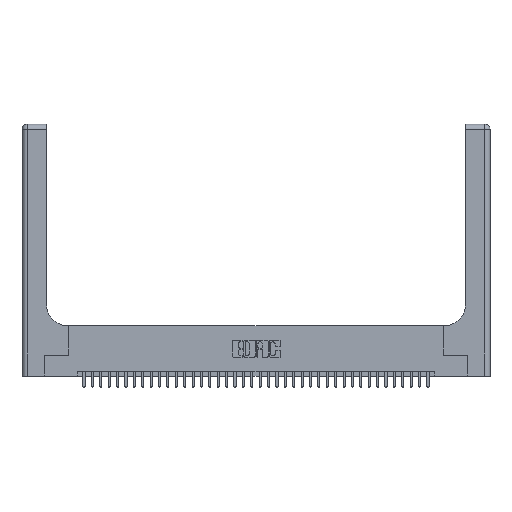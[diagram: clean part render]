
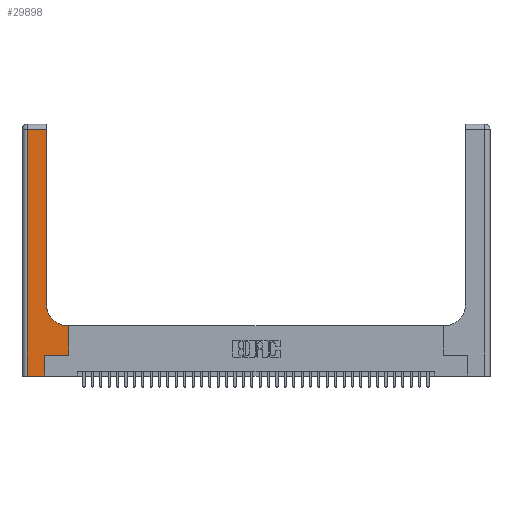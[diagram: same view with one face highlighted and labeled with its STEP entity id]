
A CAD part, top view. The second image highlights one B-rep face of the part: STEP entity #29898.
In plain terms, the highlighted planar face has unit normal (0, 0, 1).
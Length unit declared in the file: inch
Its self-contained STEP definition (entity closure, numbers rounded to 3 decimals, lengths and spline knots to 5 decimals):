
#267 = ORIENTED_EDGE ( 'NONE', *, *, #32464, .T. ) ;
#625 = DIRECTION ( 'NONE',  ( 0., -1., 0. ) ) ;
#707 = VERTEX_POINT ( 'NONE', #28314 ) ;
#1085 = LINE ( 'NONE', #29768, #14064 ) ;
#2202 = CARTESIAN_POINT ( 'NONE',  ( 0.2915, 3., 0.37 ) ) ;
#2213 = DIRECTION ( 'NONE',  ( -1., 0., 0. ) ) ;
#2572 = AXIS2_PLACEMENT_3D ( 'NONE', #37485, #19864, #2213 ) ;
#3035 = VECTOR ( 'NONE', #11251, 39.37008 ) ;
#3456 = LINE ( 'NONE', #30821, #24136 ) ;
#3548 = LINE ( 'NONE', #33597, #28807 ) ;
#3603 = VERTEX_POINT ( 'NONE', #14935 ) ;
#3703 = AXIS2_PLACEMENT_3D ( 'NONE', #13306, #33821, #16253 ) ;
#4311 = CARTESIAN_POINT ( 'NONE',  ( 0.269, 0., 0.37 ) ) ;
#5079 = EDGE_CURVE ( 'NONE', #17319, #26706, #3456, .T. ) ;
#5212 = DIRECTION ( 'NONE',  ( 0., 1., 0. ) ) ;
#5476 = ORIENTED_EDGE ( 'NONE', *, *, #27689, .T. ) ;
#7870 = LINE ( 'NONE', #21252, #30346 ) ;
#9559 = ORIENTED_EDGE ( 'NONE', *, *, #33036, .T. ) ;
#10577 = DIRECTION ( 'NONE',  ( 1., 0., 0. ) ) ;
#11113 = VERTEX_POINT ( 'NONE', #31194 ) ;
#11251 = DIRECTION ( 'NONE',  ( -1., 0., 0. ) ) ;
#12202 = VERTEX_POINT ( 'NONE', #25730 ) ;
#12264 = VERTEX_POINT ( 'NONE', #17301 ) ;
#13306 = CARTESIAN_POINT ( 'NONE',  ( 0.5415, 0.85, 0.37 ) ) ;
#14064 = VECTOR ( 'NONE', #15214, 39.37008 ) ;
#14437 = CARTESIAN_POINT ( 'NONE',  ( 0.06, 0., 0.37 ) ) ;
#14837 = EDGE_CURVE ( 'NONE', #19416, #22177, #33388, .T. ) ;
#14935 = CARTESIAN_POINT ( 'NONE',  ( 0.5585, 0.6, 0.37 ) ) ;
#15214 = DIRECTION ( 'NONE',  ( -1., 0., 0. ) ) ;
#15596 = VECTOR ( 'NONE', #15685, 39.37008 ) ;
#15685 = DIRECTION ( 'NONE',  ( 0., 1., 0. ) ) ;
#16253 = DIRECTION ( 'NONE',  ( 1., 0., 0. ) ) ;
#16588 = EDGE_CURVE ( 'NONE', #707, #19416, #37351, .T. ) ;
#16941 = PLANE ( 'NONE',  #2572 ) ;
#17301 = CARTESIAN_POINT ( 'NONE',  ( 0.269, 0.25, 0.37 ) ) ;
#17319 = VERTEX_POINT ( 'NONE', #14437 ) ;
#18132 = EDGE_CURVE ( 'NONE', #12202, #707, #29804, .T. ) ;
#18505 = CARTESIAN_POINT ( 'NONE',  ( 0.5585, 0.25, 0.37 ) ) ;
#18784 = ORIENTED_EDGE ( 'NONE', *, *, #37670, .T. ) ;
#19326 = CARTESIAN_POINT ( 'NONE',  ( 0.269, 0.25, 0.37 ) ) ;
#19416 = VERTEX_POINT ( 'NONE', #27663 ) ;
#19864 = DIRECTION ( 'NONE',  ( 0., 0., -1. ) ) ;
#21252 = CARTESIAN_POINT ( 'NONE',  ( 0.06, 3., 0.37 ) ) ;
#21465 = ORIENTED_EDGE ( 'NONE', *, *, #5079, .T. ) ;
#22177 = VERTEX_POINT ( 'NONE', #37873 ) ;
#23357 = LINE ( 'NONE', #18505, #15596 ) ;
#23522 = VECTOR ( 'NONE', #5212, 39.37008 ) ;
#24136 = VECTOR ( 'NONE', #27965, 39.37008 ) ;
#25730 = CARTESIAN_POINT ( 'NONE',  ( 0.5415, 0.6, 0.37 ) ) ;
#26331 = EDGE_LOOP ( 'NONE', ( #28880, #33809, #27396, #21465, #267, #9559, #18784, #5476, #35522 ) ) ;
#26706 = VERTEX_POINT ( 'NONE', #4311 ) ;
#27396 = ORIENTED_EDGE ( 'NONE', *, *, #36516, .T. ) ;
#27663 = CARTESIAN_POINT ( 'NONE',  ( 0.2915, 2.94, 0.37 ) ) ;
#27689 = EDGE_CURVE ( 'NONE', #3603, #12202, #1085, .T. ) ;
#27965 = DIRECTION ( 'NONE',  ( 1., 0., 0. ) ) ;
#28314 = CARTESIAN_POINT ( 'NONE',  ( 0.2915, 0.85, 0.37 ) ) ;
#28807 = VECTOR ( 'NONE', #36570, 39.37008 ) ;
#28880 = ORIENTED_EDGE ( 'NONE', *, *, #16588, .T. ) ;
#29768 = CARTESIAN_POINT ( 'NONE',  ( 0.2915, 0.6, 0.37 ) ) ;
#29804 = CIRCLE ( 'NONE', #3703, 0.25 ) ;
#29898 = ADVANCED_FACE ( 'NONE', ( #36831 ), #16941, .F. ) ;
#30148 = VECTOR ( 'NONE', #10577, 39.37008 ) ;
#30346 = VECTOR ( 'NONE', #625, 39.37008 ) ;
#30821 = CARTESIAN_POINT ( 'NONE',  ( 0., 0., 0.37 ) ) ;
#31194 = CARTESIAN_POINT ( 'NONE',  ( 0.5585, 0.25, 0.37 ) ) ;
#31774 = CARTESIAN_POINT ( 'NONE',  ( 0., 2.94, 0.37 ) ) ;
#32464 = EDGE_CURVE ( 'NONE', #26706, #12264, #3548, .T. ) ;
#33036 = EDGE_CURVE ( 'NONE', #12264, #11113, #38022, .T. ) ;
#33388 = LINE ( 'NONE', #31774, #3035 ) ;
#33597 = CARTESIAN_POINT ( 'NONE',  ( 0.269, 0., 0.37 ) ) ;
#33809 = ORIENTED_EDGE ( 'NONE', *, *, #14837, .T. ) ;
#33821 = DIRECTION ( 'NONE',  ( 0., 0., -1. ) ) ;
#35522 = ORIENTED_EDGE ( 'NONE', *, *, #18132, .T. ) ;
#36516 = EDGE_CURVE ( 'NONE', #22177, #17319, #7870, .T. ) ;
#36570 = DIRECTION ( 'NONE',  ( 0., 1., 0. ) ) ;
#36831 = FACE_OUTER_BOUND ( 'NONE', #26331, .T. ) ;
#37351 = LINE ( 'NONE', #2202, #23522 ) ;
#37485 = CARTESIAN_POINT ( 'NONE',  ( 0., 3., 0.37 ) ) ;
#37670 = EDGE_CURVE ( 'NONE', #11113, #3603, #23357, .T. ) ;
#37873 = CARTESIAN_POINT ( 'NONE',  ( 0.06, 2.94, 0.37 ) ) ;
#38022 = LINE ( 'NONE', #19326, #30148 ) ;
